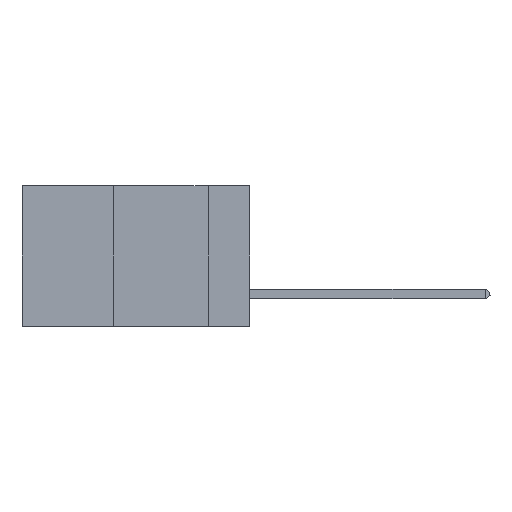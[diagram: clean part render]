
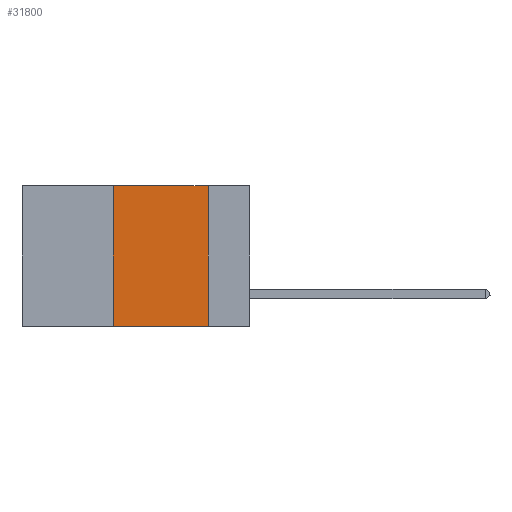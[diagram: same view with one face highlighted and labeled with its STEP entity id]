
A CAD part, left-side view. The second image highlights one B-rep face of the part: STEP entity #31800.
In plain terms, the highlighted planar face has unit normal (-1, 0, 0).
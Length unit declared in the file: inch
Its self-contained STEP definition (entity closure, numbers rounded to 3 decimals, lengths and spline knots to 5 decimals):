
#1767 = DIRECTION ( 'NONE',  ( 0., 0., -1. ) ) ;
#1949 = VERTEX_POINT ( 'NONE', #21317 ) ;
#2291 = VECTOR ( 'NONE', #32878, 39.37008 ) ;
#3074 = EDGE_CURVE ( 'NONE', #1949, #15518, #26162, .T. ) ;
#4028 = CARTESIAN_POINT ( 'NONE',  ( 0., 0.36, 0. ) ) ;
#4473 = DIRECTION ( 'NONE',  ( 0., -1., 0. ) ) ;
#7587 = VERTEX_POINT ( 'NONE', #30726 ) ;
#9374 = CARTESIAN_POINT ( 'NONE',  ( 0., 0.36, -0.37 ) ) ;
#9613 = ORIENTED_EDGE ( 'NONE', *, *, #12521, .F. ) ;
#10004 = LINE ( 'NONE', #4028, #22813 ) ;
#12507 = FACE_OUTER_BOUND ( 'NONE', #24863, .T. ) ;
#12521 = EDGE_CURVE ( 'NONE', #15518, #7587, #36850, .T. ) ;
#13639 = ORIENTED_EDGE ( 'NONE', *, *, #3074, .F. ) ;
#14147 = ORIENTED_EDGE ( 'NONE', *, *, #18250, .T. ) ;
#15518 = VERTEX_POINT ( 'NONE', #25624 ) ;
#17584 = VECTOR ( 'NONE', #4473, 39.37008 ) ;
#18250 = EDGE_CURVE ( 'NONE', #22576, #7587, #29381, .T. ) ;
#21317 = CARTESIAN_POINT ( 'NONE',  ( 0., 0.36, 0. ) ) ;
#21350 = CARTESIAN_POINT ( 'NONE',  ( 0., 0.11, 0. ) ) ;
#21411 = CARTESIAN_POINT ( 'NONE',  ( 0., 0.6, 0. ) ) ;
#22576 = VERTEX_POINT ( 'NONE', #9374 ) ;
#22813 = VECTOR ( 'NONE', #28849, 39.37008 ) ;
#24863 = EDGE_LOOP ( 'NONE', ( #9613, #13639, #27304, #14147 ) ) ;
#24929 = PLANE ( 'NONE',  #35929 ) ;
#25624 = CARTESIAN_POINT ( 'NONE',  ( 0., 0.11, 0. ) ) ;
#26162 = LINE ( 'NONE', #32771, #17584 ) ;
#27304 = ORIENTED_EDGE ( 'NONE', *, *, #34213, .F. ) ;
#27384 = VECTOR ( 'NONE', #1767, 39.37008 ) ;
#28849 = DIRECTION ( 'NONE',  ( 0., 0., 1. ) ) ;
#29160 = CARTESIAN_POINT ( 'NONE',  ( 0., 0.6, -0.37 ) ) ;
#29381 = LINE ( 'NONE', #29160, #2291 ) ;
#30726 = CARTESIAN_POINT ( 'NONE',  ( 0., 0.11, -0.37 ) ) ;
#31800 = ADVANCED_FACE ( 'NONE', ( #12507 ), #24929, .F. ) ;
#32771 = CARTESIAN_POINT ( 'NONE',  ( 0., 0.6, 0. ) ) ;
#32878 = DIRECTION ( 'NONE',  ( 0., -1., 0. ) ) ;
#34213 = EDGE_CURVE ( 'NONE', #22576, #1949, #10004, .T. ) ;
#34216 = DIRECTION ( 'NONE',  ( 0., 0., -1. ) ) ;
#35929 = AXIS2_PLACEMENT_3D ( 'NONE', #21411, #40844, #34216 ) ;
#36850 = LINE ( 'NONE', #21350, #27384 ) ;
#40844 = DIRECTION ( 'NONE',  ( 1., 0., 0. ) ) ;
